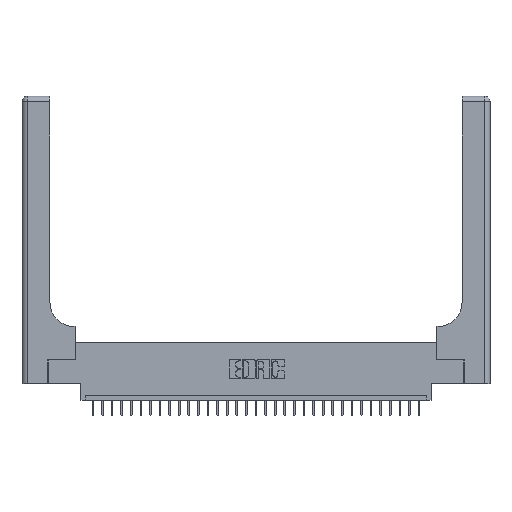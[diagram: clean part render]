
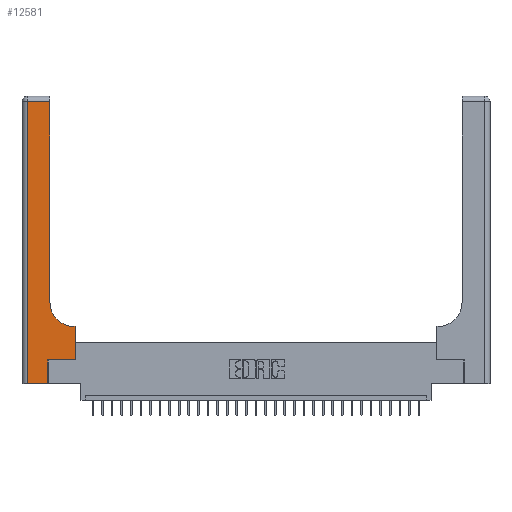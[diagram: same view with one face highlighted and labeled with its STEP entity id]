
A CAD part, top view. The second image highlights one B-rep face of the part: STEP entity #12581.
In plain terms, the highlighted planar face has unit normal (0, 0, 1).
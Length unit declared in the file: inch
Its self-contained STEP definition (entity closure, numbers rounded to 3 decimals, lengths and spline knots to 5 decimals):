
#340 = ORIENTED_EDGE ( 'NONE', *, *, #474, .T. ) ;
#474 = EDGE_CURVE ( 'NONE', #10596, #21978, #15160, .T. ) ;
#972 = VERTEX_POINT ( 'NONE', #3404 ) ;
#1026 = EDGE_CURVE ( 'NONE', #7142, #10361, #32510, .T. ) ;
#1064 = FACE_OUTER_BOUND ( 'NONE', #15242, .T. ) ;
#1536 = ORIENTED_EDGE ( 'NONE', *, *, #1026, .T. ) ;
#1728 = CARTESIAN_POINT ( 'NONE',  ( 0., 0., 0.37 ) ) ;
#1879 = CARTESIAN_POINT ( 'NONE',  ( 0.269, 0., 0.37 ) ) ;
#1961 = LINE ( 'NONE', #11343, #24845 ) ;
#2109 = DIRECTION ( 'NONE',  ( 1., 0., 0. ) ) ;
#3053 = VECTOR ( 'NONE', #31227, 39.37008 ) ;
#3069 = VECTOR ( 'NONE', #27888, 39.37008 ) ;
#3404 = CARTESIAN_POINT ( 'NONE',  ( 0.2915, 2.94, 0.37 ) ) ;
#3625 = EDGE_CURVE ( 'NONE', #10361, #20698, #1961, .T. ) ;
#4936 = ORIENTED_EDGE ( 'NONE', *, *, #6313, .T. ) ;
#4949 = CARTESIAN_POINT ( 'NONE',  ( 0.269, 0.25, 0.37 ) ) ;
#5627 = VERTEX_POINT ( 'NONE', #1879 ) ;
#5796 = AXIS2_PLACEMENT_3D ( 'NONE', #30218, #14704, #2109 ) ;
#6287 = CARTESIAN_POINT ( 'NONE',  ( 0., 3., 0.37 ) ) ;
#6313 = EDGE_CURVE ( 'NONE', #15655, #5627, #25158, .T. ) ;
#6545 = ORIENTED_EDGE ( 'NONE', *, *, #8523, .T. ) ;
#6952 = VECTOR ( 'NONE', #10427, 39.37008 ) ;
#7142 = VERTEX_POINT ( 'NONE', #4949 ) ;
#7230 = LINE ( 'NONE', #18100, #13173 ) ;
#8326 = AXIS2_PLACEMENT_3D ( 'NONE', #6287, #8954, #31567 ) ;
#8523 = EDGE_CURVE ( 'NONE', #20698, #10596, #14771, .T. ) ;
#8954 = DIRECTION ( 'NONE',  ( 0., 0., -1. ) ) ;
#10361 = VERTEX_POINT ( 'NONE', #16277 ) ;
#10427 = DIRECTION ( 'NONE',  ( 1., 0., 0. ) ) ;
#10475 = DIRECTION ( 'NONE',  ( -1., 0., 0. ) ) ;
#10524 = LINE ( 'NONE', #24474, #21173 ) ;
#10596 = VERTEX_POINT ( 'NONE', #19427 ) ;
#10725 = CARTESIAN_POINT ( 'NONE',  ( 0.5585, 0.6, 0.37 ) ) ;
#11343 = CARTESIAN_POINT ( 'NONE',  ( 0.5585, 0.25, 0.37 ) ) ;
#12457 = CARTESIAN_POINT ( 'NONE',  ( 0.2915, 3., 0.37 ) ) ;
#12581 = ADVANCED_FACE ( 'NONE', ( #1064 ), #21385, .F. ) ;
#13167 = VECTOR ( 'NONE', #30110, 39.37008 ) ;
#13173 = VECTOR ( 'NONE', #10475, 39.37008 ) ;
#13614 = VECTOR ( 'NONE', #17318, 39.37008 ) ;
#14704 = DIRECTION ( 'NONE',  ( 0., 0., -1. ) ) ;
#14740 = EDGE_CURVE ( 'NONE', #20816, #15655, #28283, .T. ) ;
#14771 = LINE ( 'NONE', #22060, #13167 ) ;
#14808 = DIRECTION ( 'NONE',  ( 0., 1., 0. ) ) ;
#15160 = CIRCLE ( 'NONE', #5796, 0.25 ) ;
#15242 = EDGE_LOOP ( 'NONE', ( #17004, #31546, #28686, #4936, #25466, #1536, #17080, #6545, #340 ) ) ;
#15655 = VERTEX_POINT ( 'NONE', #22336 ) ;
#16093 = DIRECTION ( 'NONE',  ( 0., 1., 0. ) ) ;
#16277 = CARTESIAN_POINT ( 'NONE',  ( 0.5585, 0.25, 0.37 ) ) ;
#17004 = ORIENTED_EDGE ( 'NONE', *, *, #21010, .T. ) ;
#17080 = ORIENTED_EDGE ( 'NONE', *, *, #3625, .T. ) ;
#17318 = DIRECTION ( 'NONE',  ( 1., 0., 0. ) ) ;
#18100 = CARTESIAN_POINT ( 'NONE',  ( 0., 2.94, 0.37 ) ) ;
#19036 = CARTESIAN_POINT ( 'NONE',  ( 0.06, 2.94, 0.37 ) ) ;
#19427 = CARTESIAN_POINT ( 'NONE',  ( 0.5415, 0.6, 0.37 ) ) ;
#20698 = VERTEX_POINT ( 'NONE', #10725 ) ;
#20816 = VERTEX_POINT ( 'NONE', #19036 ) ;
#20972 = EDGE_CURVE ( 'NONE', #5627, #7142, #10524, .T. ) ;
#21010 = EDGE_CURVE ( 'NONE', #21978, #972, #26335, .T. ) ;
#21173 = VECTOR ( 'NONE', #14808, 39.37008 ) ;
#21385 = PLANE ( 'NONE',  #8326 ) ;
#21978 = VERTEX_POINT ( 'NONE', #31682 ) ;
#22060 = CARTESIAN_POINT ( 'NONE',  ( 0.2915, 0.6, 0.37 ) ) ;
#22336 = CARTESIAN_POINT ( 'NONE',  ( 0.06, 0., 0.37 ) ) ;
#24474 = CARTESIAN_POINT ( 'NONE',  ( 0.269, 0., 0.37 ) ) ;
#24845 = VECTOR ( 'NONE', #16093, 39.37008 ) ;
#25158 = LINE ( 'NONE', #1728, #6952 ) ;
#25466 = ORIENTED_EDGE ( 'NONE', *, *, #20972, .T. ) ;
#26335 = LINE ( 'NONE', #12457, #3069 ) ;
#27888 = DIRECTION ( 'NONE',  ( 0., 1., 0. ) ) ;
#28283 = LINE ( 'NONE', #28816, #3053 ) ;
#28686 = ORIENTED_EDGE ( 'NONE', *, *, #14740, .T. ) ;
#28816 = CARTESIAN_POINT ( 'NONE',  ( 0.06, 3., 0.37 ) ) ;
#29248 = CARTESIAN_POINT ( 'NONE',  ( 0.269, 0.25, 0.37 ) ) ;
#30110 = DIRECTION ( 'NONE',  ( -1., 0., 0. ) ) ;
#30218 = CARTESIAN_POINT ( 'NONE',  ( 0.5415, 0.85, 0.37 ) ) ;
#30854 = EDGE_CURVE ( 'NONE', #972, #20816, #7230, .T. ) ;
#31227 = DIRECTION ( 'NONE',  ( 0., -1., 0. ) ) ;
#31546 = ORIENTED_EDGE ( 'NONE', *, *, #30854, .T. ) ;
#31567 = DIRECTION ( 'NONE',  ( -1., 0., 0. ) ) ;
#31682 = CARTESIAN_POINT ( 'NONE',  ( 0.2915, 0.85, 0.37 ) ) ;
#32510 = LINE ( 'NONE', #29248, #13614 ) ;
